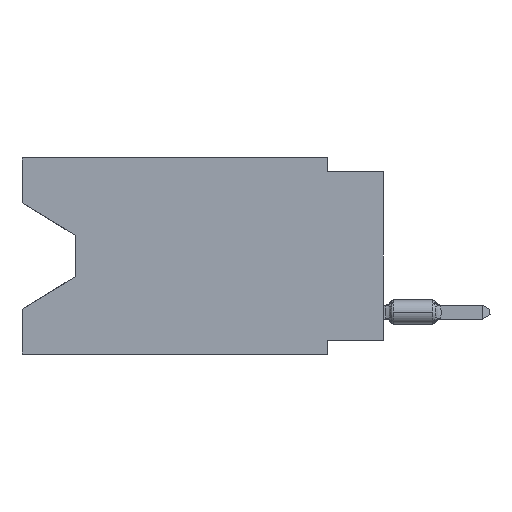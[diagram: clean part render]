
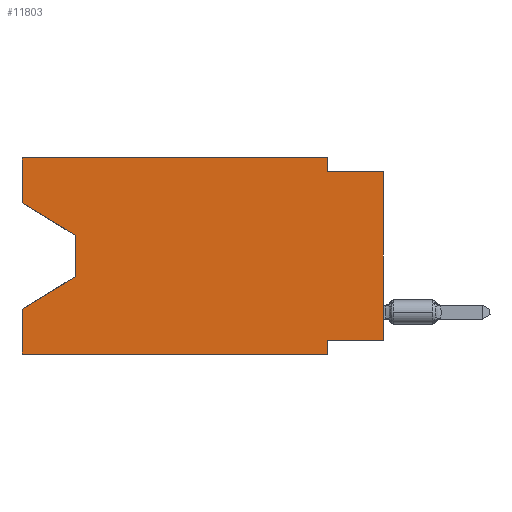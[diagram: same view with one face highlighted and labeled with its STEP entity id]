
A CAD part, left-side view. The second image highlights one B-rep face of the part: STEP entity #11803.
In plain terms, the highlighted planar face has unit normal (-1, 0, 0).
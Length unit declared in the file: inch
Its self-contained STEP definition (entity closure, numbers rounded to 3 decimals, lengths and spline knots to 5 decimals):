
#46 = VERTEX_POINT ( 'NONE', #31516 ) ;
#364 = LINE ( 'NONE', #19717, #15931 ) ;
#1197 = DIRECTION ( 'NONE',  ( 1., 0., 0. ) ) ;
#1449 = CARTESIAN_POINT ( 'NONE',  ( 0., 0.645, 0. ) ) ;
#1672 = DIRECTION ( 'NONE',  ( 0., 0., 1. ) ) ;
#1796 = VERTEX_POINT ( 'NONE', #5876 ) ;
#2176 = VERTEX_POINT ( 'NONE', #39926 ) ;
#2199 = VECTOR ( 'NONE', #9039, 39.37008 ) ;
#2229 = LINE ( 'NONE', #36713, #30563 ) ;
#2424 = VECTOR ( 'NONE', #30708, 39.37008 ) ;
#2838 = VERTEX_POINT ( 'NONE', #26510 ) ;
#3004 = EDGE_CURVE ( 'NONE', #35061, #37451, #5383, .T. ) ;
#3131 = EDGE_CURVE ( 'NONE', #2176, #37451, #10833, .T. ) ;
#4061 = ORIENTED_EDGE ( 'NONE', *, *, #3131, .T. ) ;
#4232 = VECTOR ( 'NONE', #1672, 39.37008 ) ;
#4251 = CARTESIAN_POINT ( 'NONE',  ( 0., 0., -0.325 ) ) ;
#5175 = VECTOR ( 'NONE', #6212, 39.37008 ) ;
#5383 = LINE ( 'NONE', #35670, #4232 ) ;
#5509 = LINE ( 'NONE', #20645, #35545 ) ;
#5876 = CARTESIAN_POINT ( 'NONE',  ( 0., 0.645, -0.08025 ) ) ;
#5991 = EDGE_CURVE ( 'NONE', #16643, #2176, #2229, .T. ) ;
#6086 = DIRECTION ( 'NONE',  ( 0., 0., 1. ) ) ;
#6212 = DIRECTION ( 'NONE',  ( 0., 1., 0. ) ) ;
#7109 = EDGE_CURVE ( 'NONE', #46, #23093, #35113, .T. ) ;
#7323 = LINE ( 'NONE', #11764, #26986 ) ;
#7551 = ORIENTED_EDGE ( 'NONE', *, *, #7109, .F. ) ;
#8387 = CARTESIAN_POINT ( 'NONE',  ( 0., 0.1, -0.35 ) ) ;
#9039 = DIRECTION ( 'NONE',  ( 0., -1., 0. ) ) ;
#10358 = ORIENTED_EDGE ( 'NONE', *, *, #11043, .T. ) ;
#10701 = DIRECTION ( 'NONE',  ( 0., -1., 0. ) ) ;
#10833 = LINE ( 'NONE', #25982, #32512 ) ;
#11043 = EDGE_CURVE ( 'NONE', #1796, #16643, #364, .T. ) ;
#11278 = DIRECTION ( 'NONE',  ( 0., 0., 1. ) ) ;
#11740 = EDGE_CURVE ( 'NONE', #31128, #23093, #7323, .T. ) ;
#11764 = CARTESIAN_POINT ( 'NONE',  ( 0., 0., 0. ) ) ;
#11803 = ADVANCED_FACE ( 'NONE', ( #34972 ), #31960, .F. ) ;
#12943 = EDGE_LOOP ( 'NONE', ( #10358, #38677, #4061, #28833, #23451, #23610, #16239, #24130, #7551, #43282, #24267, #14307 ) ) ;
#13141 = VECTOR ( 'NONE', #6086, 39.37008 ) ;
#13656 = LINE ( 'NONE', #40227, #5175 ) ;
#13851 = CARTESIAN_POINT ( 'NONE',  ( 0., 0.1, 0. ) ) ;
#13986 = CARTESIAN_POINT ( 'NONE',  ( 0., 0.645, -0.26975 ) ) ;
#14125 = LINE ( 'NONE', #17362, #32856 ) ;
#14307 = ORIENTED_EDGE ( 'NONE', *, *, #42157, .F. ) ;
#15562 = CARTESIAN_POINT ( 'NONE',  ( 0., 0.1, -0.35 ) ) ;
#15738 = DIRECTION ( 'NONE',  ( 0., -0.855, -0.519 ) ) ;
#15931 = VECTOR ( 'NONE', #15738, 39.37008 ) ;
#16239 = ORIENTED_EDGE ( 'NONE', *, *, #25437, .F. ) ;
#16482 = CARTESIAN_POINT ( 'NONE',  ( 0., 0., -0.025 ) ) ;
#16643 = VERTEX_POINT ( 'NONE', #31001 ) ;
#17362 = CARTESIAN_POINT ( 'NONE',  ( 0., 0.645, 0. ) ) ;
#18078 = LINE ( 'NONE', #13851, #22692 ) ;
#18091 = DIRECTION ( 'NONE',  ( 0., 0., -1. ) ) ;
#19717 = CARTESIAN_POINT ( 'NONE',  ( 0., 0.645, -0.08025 ) ) ;
#20645 = CARTESIAN_POINT ( 'NONE',  ( 0., 0.645, -0.35 ) ) ;
#21715 = LINE ( 'NONE', #47790, #13141 ) ;
#22692 = VECTOR ( 'NONE', #28516, 39.37008 ) ;
#23093 = VERTEX_POINT ( 'NONE', #42171 ) ;
#23451 = ORIENTED_EDGE ( 'NONE', *, *, #46516, .T. ) ;
#23610 = ORIENTED_EDGE ( 'NONE', *, *, #34395, .F. ) ;
#24130 = ORIENTED_EDGE ( 'NONE', *, *, #11740, .T. ) ;
#24267 = ORIENTED_EDGE ( 'NONE', *, *, #39079, .F. ) ;
#25064 = DIRECTION ( 'NONE',  ( 0., -1., 0. ) ) ;
#25437 = EDGE_CURVE ( 'NONE', #31128, #2838, #13656, .T. ) ;
#25982 = CARTESIAN_POINT ( 'NONE',  ( 0., 0.55, -0.212 ) ) ;
#26510 = CARTESIAN_POINT ( 'NONE',  ( 0., 0.1, -0.325 ) ) ;
#26986 = VECTOR ( 'NONE', #11278, 39.37008 ) ;
#27258 = DIRECTION ( 'NONE',  ( 0., 0., -1. ) ) ;
#27722 = LINE ( 'NONE', #15562, #2424 ) ;
#28516 = DIRECTION ( 'NONE',  ( 0., 0., -1. ) ) ;
#28833 = ORIENTED_EDGE ( 'NONE', *, *, #3004, .F. ) ;
#30414 = EDGE_CURVE ( 'NONE', #34765, #46, #18078, .T. ) ;
#30563 = VECTOR ( 'NONE', #18091, 39.37008 ) ;
#30708 = DIRECTION ( 'NONE',  ( 0., 0., -1. ) ) ;
#31001 = CARTESIAN_POINT ( 'NONE',  ( 0., 0.55, -0.138 ) ) ;
#31128 = VERTEX_POINT ( 'NONE', #4251 ) ;
#31516 = CARTESIAN_POINT ( 'NONE',  ( 0., 0.1, -0.025 ) ) ;
#31960 = PLANE ( 'NONE',  #45199 ) ;
#32512 = VECTOR ( 'NONE', #46048, 39.37008 ) ;
#32856 = VECTOR ( 'NONE', #25064, 39.37008 ) ;
#33424 = CARTESIAN_POINT ( 'NONE',  ( 0., 0.1, 0. ) ) ;
#34395 = EDGE_CURVE ( 'NONE', #2838, #40576, #27722, .T. ) ;
#34464 = CARTESIAN_POINT ( 'NONE',  ( 0., 0.645, -0.35 ) ) ;
#34765 = VERTEX_POINT ( 'NONE', #33424 ) ;
#34972 = FACE_OUTER_BOUND ( 'NONE', #12943, .T. ) ;
#35061 = VERTEX_POINT ( 'NONE', #34464 ) ;
#35113 = LINE ( 'NONE', #16482, #2199 ) ;
#35545 = VECTOR ( 'NONE', #10701, 39.37008 ) ;
#35670 = CARTESIAN_POINT ( 'NONE',  ( 0., 0.645, 0. ) ) ;
#36713 = CARTESIAN_POINT ( 'NONE',  ( 0., 0.55, -0.138 ) ) ;
#37451 = VERTEX_POINT ( 'NONE', #13986 ) ;
#38677 = ORIENTED_EDGE ( 'NONE', *, *, #5991, .T. ) ;
#39079 = EDGE_CURVE ( 'NONE', #45203, #34765, #14125, .T. ) ;
#39926 = CARTESIAN_POINT ( 'NONE',  ( 0., 0.55, -0.212 ) ) ;
#40227 = CARTESIAN_POINT ( 'NONE',  ( 0., 0., -0.325 ) ) ;
#40247 = CARTESIAN_POINT ( 'NONE',  ( 0., 0.645, 0. ) ) ;
#40576 = VERTEX_POINT ( 'NONE', #8387 ) ;
#42157 = EDGE_CURVE ( 'NONE', #1796, #45203, #21715, .T. ) ;
#42171 = CARTESIAN_POINT ( 'NONE',  ( 0., 0., -0.025 ) ) ;
#43282 = ORIENTED_EDGE ( 'NONE', *, *, #30414, .F. ) ;
#45199 = AXIS2_PLACEMENT_3D ( 'NONE', #1449, #1197, #27258 ) ;
#45203 = VERTEX_POINT ( 'NONE', #40247 ) ;
#46048 = DIRECTION ( 'NONE',  ( 0., 0.855, -0.519 ) ) ;
#46516 = EDGE_CURVE ( 'NONE', #35061, #40576, #5509, .T. ) ;
#47790 = CARTESIAN_POINT ( 'NONE',  ( 0., 0.645, 0. ) ) ;
